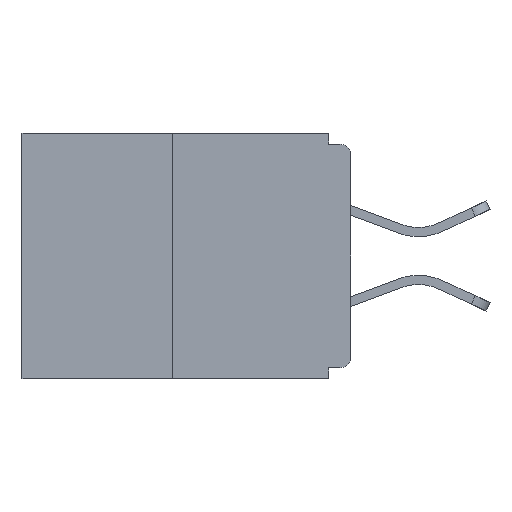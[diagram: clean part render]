
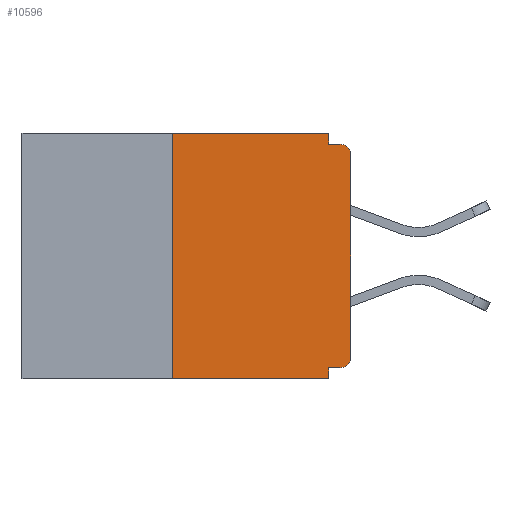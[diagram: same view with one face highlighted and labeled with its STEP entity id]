
A CAD part, left-side view. The second image highlights one B-rep face of the part: STEP entity #10596.
In plain terms, the highlighted planar face has unit normal (-1, 0, 0).
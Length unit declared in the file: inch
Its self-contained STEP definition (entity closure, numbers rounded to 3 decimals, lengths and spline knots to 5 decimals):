
#4 = DIRECTION ( 'NONE',  ( 0., 0., -1. ) ) ;
#203 = ORIENTED_EDGE ( 'NONE', *, *, #7972, .T. ) ;
#322 = DIRECTION ( 'NONE',  ( 1., 0., 0. ) ) ;
#816 = VECTOR ( 'NONE', #5640, 39.37008 ) ;
#880 = LINE ( 'NONE', #5085, #4730 ) ;
#990 = ORIENTED_EDGE ( 'NONE', *, *, #3275, .F. ) ;
#1125 = CARTESIAN_POINT ( 'NONE',  ( 0., 0.46, 0. ) ) ;
#1626 = DIRECTION ( 'NONE',  ( 0., 0., -1. ) ) ;
#1643 = CARTESIAN_POINT ( 'NONE',  ( 0., 0.031, -0.328 ) ) ;
#1740 = VERTEX_POINT ( 'NONE', #3945 ) ;
#1752 = CARTESIAN_POINT ( 'NONE',  ( 0., 0., -0.313 ) ) ;
#1825 = VERTEX_POINT ( 'NONE', #9173 ) ;
#1835 = EDGE_CURVE ( 'NONE', #1825, #1740, #880, .T. ) ;
#2069 = EDGE_CURVE ( 'NONE', #9082, #9221, #4716, .T. ) ;
#2074 = ORIENTED_EDGE ( 'NONE', *, *, #9006, .F. ) ;
#2156 = DIRECTION ( 'NONE',  ( -1., 0., 0. ) ) ;
#2193 = CARTESIAN_POINT ( 'NONE',  ( 0., 0., -0.328 ) ) ;
#2301 = CARTESIAN_POINT ( 'NONE',  ( 0., 0.031, -0.343 ) ) ;
#2329 = VECTOR ( 'NONE', #3808, 39.37008 ) ;
#2596 = EDGE_CURVE ( 'NONE', #1740, #8373, #7257, .T. ) ;
#2834 = VECTOR ( 'NONE', #6215, 39.37008 ) ;
#2851 = LINE ( 'NONE', #2193, #2329 ) ;
#2857 = CIRCLE ( 'NONE', #6885, 0.015 ) ;
#2866 = VECTOR ( 'NONE', #1626, 39.37008 ) ;
#2867 = PLANE ( 'NONE',  #9183 ) ;
#3205 = ORIENTED_EDGE ( 'NONE', *, *, #2596, .F. ) ;
#3275 = EDGE_CURVE ( 'NONE', #9082, #10928, #2851, .T. ) ;
#3580 = ORIENTED_EDGE ( 'NONE', *, *, #3799, .F. ) ;
#3799 = EDGE_CURVE ( 'NONE', #5430, #1825, #10474, .T. ) ;
#3808 = DIRECTION ( 'NONE',  ( 0., 1., 0. ) ) ;
#3922 = DIRECTION ( 'NONE',  ( 0., -1., 0. ) ) ;
#3945 = CARTESIAN_POINT ( 'NONE',  ( 0., 0.031, 0. ) ) ;
#4034 = CARTESIAN_POINT ( 'NONE',  ( 0., 0.031, 0. ) ) ;
#4223 = ORIENTED_EDGE ( 'NONE', *, *, #7988, .F. ) ;
#4283 = AXIS2_PLACEMENT_3D ( 'NONE', #10684, #2156, #9852 ) ;
#4518 = CARTESIAN_POINT ( 'NONE',  ( 0., 0.25, 0. ) ) ;
#4572 = DIRECTION ( 'NONE',  ( 0., 0., -1. ) ) ;
#4716 = CIRCLE ( 'NONE', #4283, 0.015 ) ;
#4730 = VECTOR ( 'NONE', #6780, 39.37008 ) ;
#4927 = ORIENTED_EDGE ( 'NONE', *, *, #6130, .T. ) ;
#5051 = ORIENTED_EDGE ( 'NONE', *, *, #1835, .F. ) ;
#5085 = CARTESIAN_POINT ( 'NONE',  ( 0., 0.46, 0. ) ) ;
#5087 = LINE ( 'NONE', #2301, #816 ) ;
#5430 = VERTEX_POINT ( 'NONE', #9694 ) ;
#5640 = DIRECTION ( 'NONE',  ( 0., 0., -1. ) ) ;
#5673 = CARTESIAN_POINT ( 'NONE',  ( 0., 0.46, -0.343 ) ) ;
#5747 = LINE ( 'NONE', #8591, #7886 ) ;
#6037 = CARTESIAN_POINT ( 'NONE',  ( 0., 0.015, -0.03 ) ) ;
#6084 = FACE_OUTER_BOUND ( 'NONE', #10234, .T. ) ;
#6130 = EDGE_CURVE ( 'NONE', #9221, #6336, #5747, .T. ) ;
#6183 = VERTEX_POINT ( 'NONE', #6210 ) ;
#6210 = CARTESIAN_POINT ( 'NONE',  ( 0., 0.031, -0.343 ) ) ;
#6215 = DIRECTION ( 'NONE',  ( 0., 0., 1. ) ) ;
#6336 = VERTEX_POINT ( 'NONE', #7712 ) ;
#6630 = LINE ( 'NONE', #5673, #10673 ) ;
#6780 = DIRECTION ( 'NONE',  ( 0., -1., 0. ) ) ;
#6885 = AXIS2_PLACEMENT_3D ( 'NONE', #6037, #8664, #4 ) ;
#7257 = LINE ( 'NONE', #4034, #2866 ) ;
#7712 = CARTESIAN_POINT ( 'NONE',  ( 0., 0., -0.03 ) ) ;
#7886 = VECTOR ( 'NONE', #10449, 39.37008 ) ;
#7972 = EDGE_CURVE ( 'NONE', #6336, #8336, #2857, .T. ) ;
#7988 = EDGE_CURVE ( 'NONE', #8373, #8336, #8851, .T. ) ;
#8308 = VECTOR ( 'NONE', #8586, 39.37008 ) ;
#8336 = VERTEX_POINT ( 'NONE', #10064 ) ;
#8373 = VERTEX_POINT ( 'NONE', #9056 ) ;
#8519 = CARTESIAN_POINT ( 'NONE',  ( 0., 0., -0.015 ) ) ;
#8586 = DIRECTION ( 'NONE',  ( 0., -1., 0. ) ) ;
#8591 = CARTESIAN_POINT ( 'NONE',  ( 0., 0., 0. ) ) ;
#8664 = DIRECTION ( 'NONE',  ( -1., 0., 0. ) ) ;
#8851 = LINE ( 'NONE', #8519, #8308 ) ;
#9006 = EDGE_CURVE ( 'NONE', #10928, #6183, #5087, .T. ) ;
#9056 = CARTESIAN_POINT ( 'NONE',  ( 0., 0.031, -0.015 ) ) ;
#9082 = VERTEX_POINT ( 'NONE', #10874 ) ;
#9173 = CARTESIAN_POINT ( 'NONE',  ( 0., 0.25, 0. ) ) ;
#9183 = AXIS2_PLACEMENT_3D ( 'NONE', #1125, #322, #4572 ) ;
#9221 = VERTEX_POINT ( 'NONE', #1752 ) ;
#9313 = ORIENTED_EDGE ( 'NONE', *, *, #2069, .T. ) ;
#9694 = CARTESIAN_POINT ( 'NONE',  ( 0., 0.25, -0.343 ) ) ;
#9852 = DIRECTION ( 'NONE',  ( 0., 0., -1. ) ) ;
#9987 = ORIENTED_EDGE ( 'NONE', *, *, #10195, .T. ) ;
#10064 = CARTESIAN_POINT ( 'NONE',  ( 0., 0.015, -0.015 ) ) ;
#10195 = EDGE_CURVE ( 'NONE', #5430, #6183, #6630, .T. ) ;
#10234 = EDGE_LOOP ( 'NONE', ( #5051, #3580, #9987, #2074, #990, #9313, #4927, #203, #4223, #3205 ) ) ;
#10449 = DIRECTION ( 'NONE',  ( 0., 0., 1. ) ) ;
#10474 = LINE ( 'NONE', #4518, #2834 ) ;
#10596 = ADVANCED_FACE ( 'NONE', ( #6084 ), #2867, .F. ) ;
#10673 = VECTOR ( 'NONE', #3922, 39.37008 ) ;
#10684 = CARTESIAN_POINT ( 'NONE',  ( 0., 0.015, -0.313 ) ) ;
#10874 = CARTESIAN_POINT ( 'NONE',  ( 0., 0.015, -0.328 ) ) ;
#10928 = VERTEX_POINT ( 'NONE', #1643 ) ;
